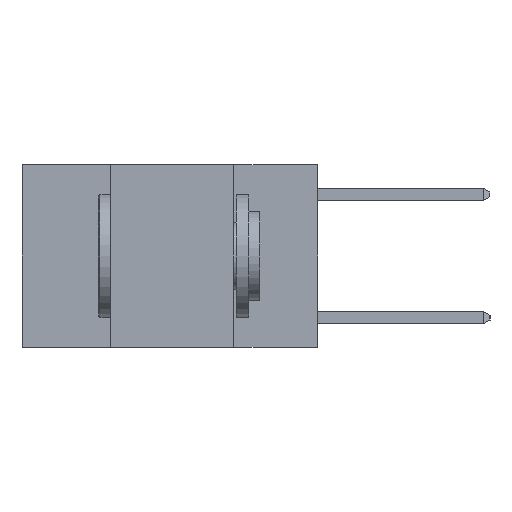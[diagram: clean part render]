
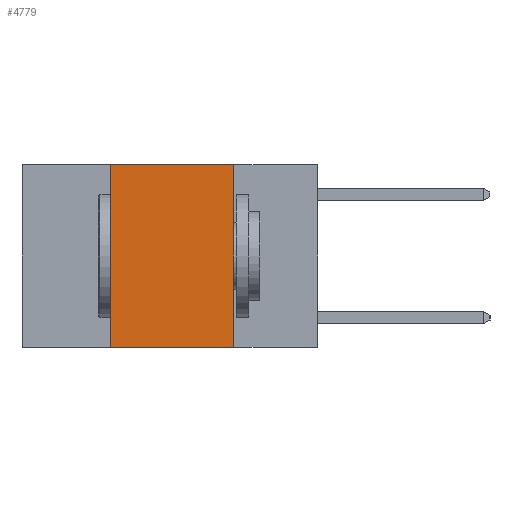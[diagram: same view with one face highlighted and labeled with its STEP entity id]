
A CAD part, left-side view. The second image highlights one B-rep face of the part: STEP entity #4779.
In plain terms, the highlighted planar face has unit normal (-1, 0, 0).
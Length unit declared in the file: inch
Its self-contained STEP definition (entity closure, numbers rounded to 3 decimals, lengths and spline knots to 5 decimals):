
#276 = PLANE ( 'NONE',  #2487 ) ;
#358 = LINE ( 'NONE', #6459, #9180 ) ;
#391 = CARTESIAN_POINT ( 'NONE',  ( 0., 0.42, 0. ) ) ;
#897 = CARTESIAN_POINT ( 'NONE',  ( 0., 0.42, -0.37 ) ) ;
#966 = EDGE_LOOP ( 'NONE', ( #7811, #2722, #2812, #5900 ) ) ;
#1338 = DIRECTION ( 'NONE',  ( 0., -1., 0. ) ) ;
#1401 = VERTEX_POINT ( 'NONE', #8022 ) ;
#2174 = CARTESIAN_POINT ( 'NONE',  ( 0., 0.6, 0. ) ) ;
#2487 = AXIS2_PLACEMENT_3D ( 'NONE', #2174, #3918, #9953 ) ;
#2722 = ORIENTED_EDGE ( 'NONE', *, *, #2965, .F. ) ;
#2812 = ORIENTED_EDGE ( 'NONE', *, *, #8692, .F. ) ;
#2889 = EDGE_CURVE ( 'NONE', #9028, #3188, #11058, .T. ) ;
#2965 = EDGE_CURVE ( 'NONE', #1401, #3255, #9999, .T. ) ;
#3188 = VERTEX_POINT ( 'NONE', #4252 ) ;
#3255 = VERTEX_POINT ( 'NONE', #4384 ) ;
#3594 = FACE_OUTER_BOUND ( 'NONE', #966, .T. ) ;
#3918 = DIRECTION ( 'NONE',  ( 1., 0., 0. ) ) ;
#4252 = CARTESIAN_POINT ( 'NONE',  ( 0., 0.17, -0.37 ) ) ;
#4384 = CARTESIAN_POINT ( 'NONE',  ( 0., 0.17, 0. ) ) ;
#4475 = VECTOR ( 'NONE', #10050, 39.37008 ) ;
#4779 = ADVANCED_FACE ( 'NONE', ( #3594 ), #276, .F. ) ;
#5606 = DIRECTION ( 'NONE',  ( 0., 0., -1. ) ) ;
#5608 = CARTESIAN_POINT ( 'NONE',  ( 0., 0.6, -0.37 ) ) ;
#5900 = ORIENTED_EDGE ( 'NONE', *, *, #2889, .T. ) ;
#6459 = CARTESIAN_POINT ( 'NONE',  ( 0., 0.17, 0. ) ) ;
#6763 = LINE ( 'NONE', #391, #4475 ) ;
#7313 = DIRECTION ( 'NONE',  ( 0., -1., 0. ) ) ;
#7421 = CARTESIAN_POINT ( 'NONE',  ( 0., 0.6, 0. ) ) ;
#7811 = ORIENTED_EDGE ( 'NONE', *, *, #9835, .F. ) ;
#8022 = CARTESIAN_POINT ( 'NONE',  ( 0., 0.42, 0. ) ) ;
#8521 = VECTOR ( 'NONE', #7313, 39.37008 ) ;
#8692 = EDGE_CURVE ( 'NONE', #9028, #1401, #6763, .T. ) ;
#9028 = VERTEX_POINT ( 'NONE', #897 ) ;
#9180 = VECTOR ( 'NONE', #5606, 39.37008 ) ;
#9835 = EDGE_CURVE ( 'NONE', #3255, #3188, #358, .T. ) ;
#9953 = DIRECTION ( 'NONE',  ( 0., 0., -1. ) ) ;
#9999 = LINE ( 'NONE', #7421, #10256 ) ;
#10050 = DIRECTION ( 'NONE',  ( 0., 0., 1. ) ) ;
#10256 = VECTOR ( 'NONE', #1338, 39.37008 ) ;
#11058 = LINE ( 'NONE', #5608, #8521 ) ;
